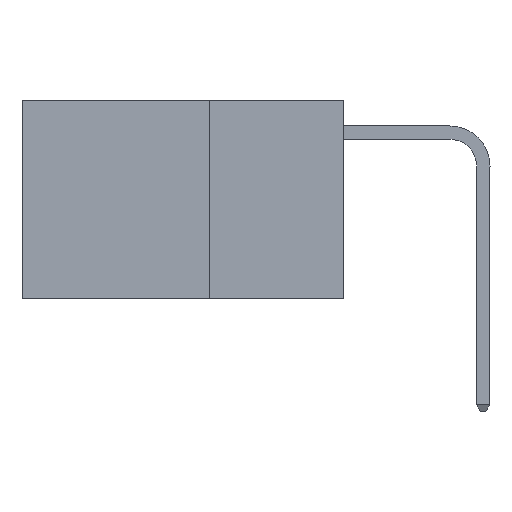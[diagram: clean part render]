
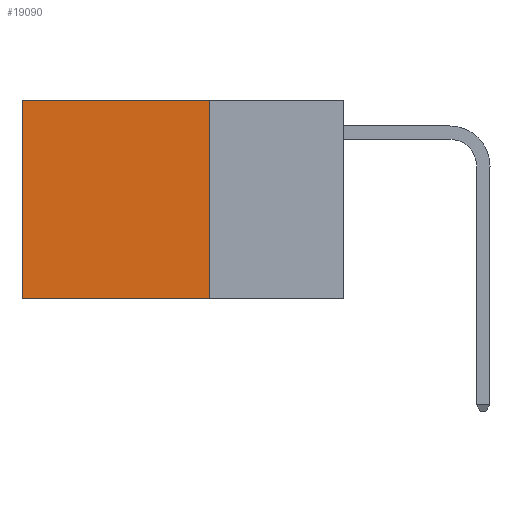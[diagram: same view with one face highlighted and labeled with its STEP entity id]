
A CAD part, left-side view. The second image highlights one B-rep face of the part: STEP entity #19090.
In plain terms, the highlighted planar face has unit normal (-1, 0, 0).
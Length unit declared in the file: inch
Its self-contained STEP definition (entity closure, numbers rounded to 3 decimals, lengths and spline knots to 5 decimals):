
#352 = DIRECTION ( 'NONE',  ( 0., 0., -1. ) ) ;
#1057 = ORIENTED_EDGE ( 'NONE', *, *, #10948, .T. ) ;
#1554 = PLANE ( 'NONE',  #4479 ) ;
#2110 = ORIENTED_EDGE ( 'NONE', *, *, #16676, .F. ) ;
#2591 = ORIENTED_EDGE ( 'NONE', *, *, #21305, .F. ) ;
#3281 = DIRECTION ( 'NONE',  ( 1., 0., 0. ) ) ;
#4479 = AXIS2_PLACEMENT_3D ( 'NONE', #13466, #3281, #15159 ) ;
#5829 = ORIENTED_EDGE ( 'NONE', *, *, #7488, .T. ) ;
#6767 = VECTOR ( 'NONE', #19322, 39.37008 ) ;
#7488 = EDGE_CURVE ( 'NONE', #8186, #9054, #17626, .T. ) ;
#7561 = CARTESIAN_POINT ( 'NONE',  ( 0.2625, 0.25, 0. ) ) ;
#7791 = CARTESIAN_POINT ( 'NONE',  ( 0.2625, 0.25, 0. ) ) ;
#8125 = VECTOR ( 'NONE', #352, 39.37008 ) ;
#8186 = VERTEX_POINT ( 'NONE', #13576 ) ;
#8681 = VECTOR ( 'NONE', #13450, 39.37008 ) ;
#8847 = FACE_OUTER_BOUND ( 'NONE', #15766, .T. ) ;
#9020 = CARTESIAN_POINT ( 'NONE',  ( 0.2625, 0.6, -0.37 ) ) ;
#9054 = VERTEX_POINT ( 'NONE', #9020 ) ;
#9185 = LINE ( 'NONE', #10597, #8125 ) ;
#9861 = LINE ( 'NONE', #21184, #15363 ) ;
#10597 = CARTESIAN_POINT ( 'NONE',  ( 0.2625, 0.25, 0. ) ) ;
#10948 = EDGE_CURVE ( 'NONE', #17453, #8186, #11293, .T. ) ;
#10992 = CARTESIAN_POINT ( 'NONE',  ( 0.2625, 0.25, -0.37 ) ) ;
#11293 = LINE ( 'NONE', #7561, #6767 ) ;
#12864 = DIRECTION ( 'NONE',  ( 0., 1., 0. ) ) ;
#13450 = DIRECTION ( 'NONE',  ( 0., 0., -1. ) ) ;
#13466 = CARTESIAN_POINT ( 'NONE',  ( 0.2625, 0.25, 0. ) ) ;
#13576 = CARTESIAN_POINT ( 'NONE',  ( 0.2625, 0.6, 0. ) ) ;
#14595 = VERTEX_POINT ( 'NONE', #10992 ) ;
#15159 = DIRECTION ( 'NONE',  ( 0., 0., -1. ) ) ;
#15363 = VECTOR ( 'NONE', #12864, 39.37008 ) ;
#15766 = EDGE_LOOP ( 'NONE', ( #5829, #2591, #2110, #1057 ) ) ;
#16676 = EDGE_CURVE ( 'NONE', #17453, #14595, #9185, .T. ) ;
#17453 = VERTEX_POINT ( 'NONE', #7791 ) ;
#17626 = LINE ( 'NONE', #18439, #8681 ) ;
#18439 = CARTESIAN_POINT ( 'NONE',  ( 0.2625, 0.6, 0. ) ) ;
#19090 = ADVANCED_FACE ( 'NONE', ( #8847 ), #1554, .F. ) ;
#19322 = DIRECTION ( 'NONE',  ( 0., 1., 0. ) ) ;
#21184 = CARTESIAN_POINT ( 'NONE',  ( 0.2625, 0.25, -0.37 ) ) ;
#21305 = EDGE_CURVE ( 'NONE', #14595, #9054, #9861, .T. ) ;
